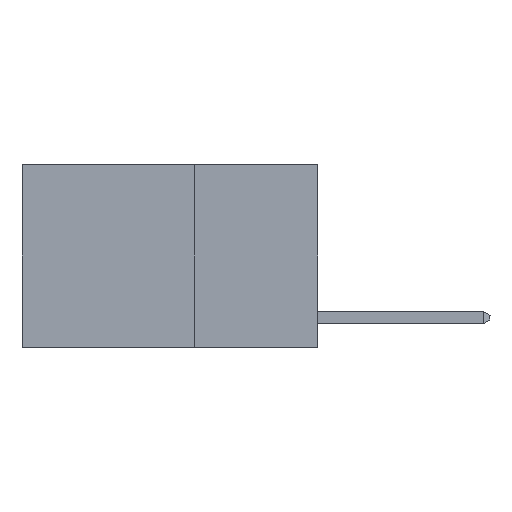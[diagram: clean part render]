
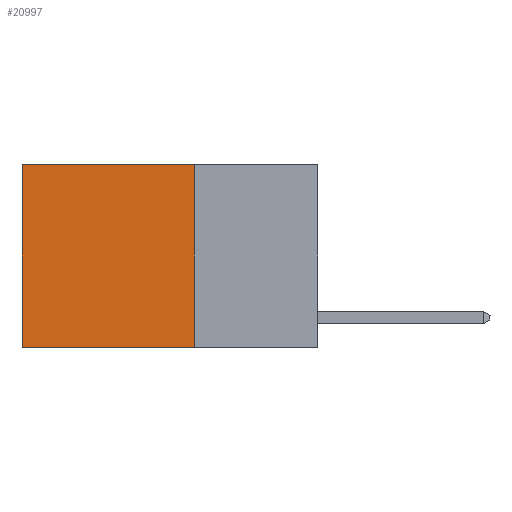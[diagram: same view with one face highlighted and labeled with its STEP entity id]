
A CAD part, left-side view. The second image highlights one B-rep face of the part: STEP entity #20997.
In plain terms, the highlighted planar face has unit normal (-1, 0, 0).
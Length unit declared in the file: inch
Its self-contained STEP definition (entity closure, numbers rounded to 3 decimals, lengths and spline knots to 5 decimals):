
#55 = VECTOR ( 'NONE', #26889, 39.37008 ) ;
#557 = PLANE ( 'NONE',  #14483 ) ;
#924 = CARTESIAN_POINT ( 'NONE',  ( 0.2625, 0.25, 0. ) ) ;
#1044 = EDGE_CURVE ( 'NONE', #4142, #3481, #27047, .T. ) ;
#1233 = VECTOR ( 'NONE', #19851, 39.37008 ) ;
#2557 = LINE ( 'NONE', #9174, #12125 ) ;
#3170 = EDGE_CURVE ( 'NONE', #4142, #20472, #17072, .T. ) ;
#3481 = VERTEX_POINT ( 'NONE', #23391 ) ;
#4142 = VERTEX_POINT ( 'NONE', #8391 ) ;
#4544 = EDGE_CURVE ( 'NONE', #3481, #20416, #27208, .T. ) ;
#4785 = DIRECTION ( 'NONE',  ( 0., 0., -1. ) ) ;
#5582 = FACE_OUTER_BOUND ( 'NONE', #16029, .T. ) ;
#7039 = ORIENTED_EDGE ( 'NONE', *, *, #1044, .T. ) ;
#8391 = CARTESIAN_POINT ( 'NONE',  ( 0.2625, 0.25, 0. ) ) ;
#8625 = CARTESIAN_POINT ( 'NONE',  ( 0.2625, 0.6, 0. ) ) ;
#8772 = ORIENTED_EDGE ( 'NONE', *, *, #3170, .F. ) ;
#9174 = CARTESIAN_POINT ( 'NONE',  ( 0.2625, 0.25, -0.37 ) ) ;
#9448 = ORIENTED_EDGE ( 'NONE', *, *, #11094, .F. ) ;
#9703 = ORIENTED_EDGE ( 'NONE', *, *, #4544, .T. ) ;
#11094 = EDGE_CURVE ( 'NONE', #20472, #20416, #2557, .T. ) ;
#11369 = VECTOR ( 'NONE', #4785, 39.37008 ) ;
#12125 = VECTOR ( 'NONE', #15662, 39.37008 ) ;
#12177 = CARTESIAN_POINT ( 'NONE',  ( 0.2625, 0.25, 0. ) ) ;
#14483 = AXIS2_PLACEMENT_3D ( 'NONE', #924, #26047, #26410 ) ;
#15437 = CARTESIAN_POINT ( 'NONE',  ( 0.2625, 0.6, -0.37 ) ) ;
#15662 = DIRECTION ( 'NONE',  ( 0., 1., 0. ) ) ;
#16029 = EDGE_LOOP ( 'NONE', ( #9703, #9448, #8772, #7039 ) ) ;
#17072 = LINE ( 'NONE', #26020, #1233 ) ;
#18132 = CARTESIAN_POINT ( 'NONE',  ( 0.2625, 0.25, -0.37 ) ) ;
#19851 = DIRECTION ( 'NONE',  ( 0., 0., -1. ) ) ;
#20416 = VERTEX_POINT ( 'NONE', #15437 ) ;
#20472 = VERTEX_POINT ( 'NONE', #18132 ) ;
#20997 = ADVANCED_FACE ( 'NONE', ( #5582 ), #557, .F. ) ;
#23391 = CARTESIAN_POINT ( 'NONE',  ( 0.2625, 0.6, 0. ) ) ;
#26020 = CARTESIAN_POINT ( 'NONE',  ( 0.2625, 0.25, 0. ) ) ;
#26047 = DIRECTION ( 'NONE',  ( 1., 0., 0. ) ) ;
#26410 = DIRECTION ( 'NONE',  ( 0., 0., -1. ) ) ;
#26889 = DIRECTION ( 'NONE',  ( 0., 1., 0. ) ) ;
#27047 = LINE ( 'NONE', #12177, #55 ) ;
#27208 = LINE ( 'NONE', #8625, #11369 ) ;
